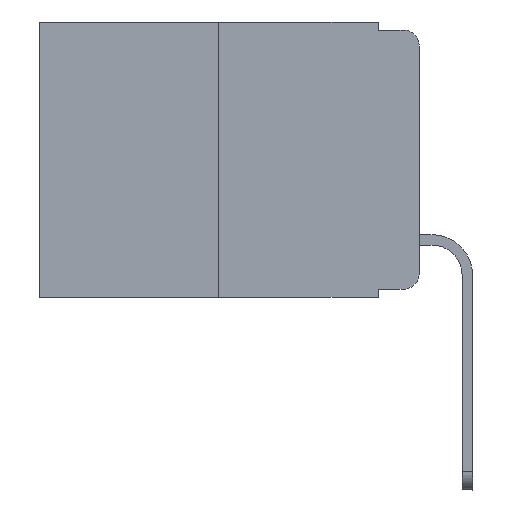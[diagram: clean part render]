
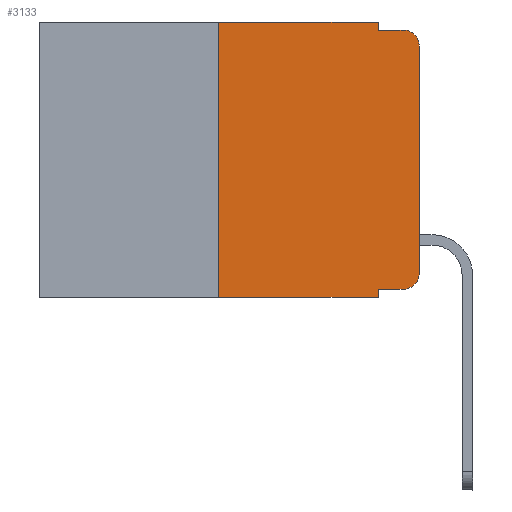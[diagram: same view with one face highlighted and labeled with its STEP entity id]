
A CAD part, left-side view. The second image highlights one B-rep face of the part: STEP entity #3133.
In plain terms, the highlighted planar face has unit normal (-1, 0, 0).
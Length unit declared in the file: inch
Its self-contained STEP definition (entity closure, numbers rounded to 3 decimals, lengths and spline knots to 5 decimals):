
#515 = DIRECTION ( 'NONE',  ( 1., 0., 0. ) ) ;
#656 = DIRECTION ( 'NONE',  ( -1., 0., 0. ) ) ;
#738 = VERTEX_POINT ( 'NONE', #8923 ) ;
#1302 = VECTOR ( 'NONE', #2873, 39.37008 ) ;
#1742 = ORIENTED_EDGE ( 'NONE', *, *, #2177, .F. ) ;
#1848 = CARTESIAN_POINT ( 'NONE',  ( 0., 0.051, 0. ) ) ;
#1941 = ORIENTED_EDGE ( 'NONE', *, *, #5974, .F. ) ;
#1996 = ORIENTED_EDGE ( 'NONE', *, *, #6174, .F. ) ;
#2177 = EDGE_CURVE ( 'NONE', #8845, #738, #9205, .T. ) ;
#2179 = CARTESIAN_POINT ( 'NONE',  ( 0., 0.25, -0.343 ) ) ;
#2196 = EDGE_CURVE ( 'NONE', #9051, #10114, #7529, .T. ) ;
#2361 = CARTESIAN_POINT ( 'NONE',  ( 0., 0.25, 0. ) ) ;
#2462 = AXIS2_PLACEMENT_3D ( 'NONE', #6807, #656, #8802 ) ;
#2551 = ORIENTED_EDGE ( 'NONE', *, *, #8033, .F. ) ;
#2873 = DIRECTION ( 'NONE',  ( 0., -1., 0. ) ) ;
#3044 = EDGE_CURVE ( 'NONE', #10114, #738, #8466, .T. ) ;
#3133 = ADVANCED_FACE ( 'NONE', ( #9075 ), #5826, .F. ) ;
#3138 = VERTEX_POINT ( 'NONE', #8938 ) ;
#3231 = VERTEX_POINT ( 'NONE', #10096 ) ;
#3804 = VERTEX_POINT ( 'NONE', #2179 ) ;
#4222 = CARTESIAN_POINT ( 'NONE',  ( 0., 0.02, -0.313 ) ) ;
#4401 = DIRECTION ( 'NONE',  ( 0., 0., 1. ) ) ;
#4646 = ORIENTED_EDGE ( 'NONE', *, *, #10714, .T. ) ;
#5015 = VERTEX_POINT ( 'NONE', #7576 ) ;
#5165 = DIRECTION ( 'NONE',  ( 0., 0., -1. ) ) ;
#5441 = VECTOR ( 'NONE', #5165, 39.37008 ) ;
#5453 = VECTOR ( 'NONE', #4401, 39.37008 ) ;
#5532 = CARTESIAN_POINT ( 'NONE',  ( 0., 0.051, -0.333 ) ) ;
#5826 = PLANE ( 'NONE',  #11360 ) ;
#5919 = LINE ( 'NONE', #10426, #5441 ) ;
#5974 = EDGE_CURVE ( 'NONE', #7213, #3231, #6970, .T. ) ;
#6174 = EDGE_CURVE ( 'NONE', #5015, #6857, #5919, .T. ) ;
#6487 = CARTESIAN_POINT ( 'NONE',  ( 0., 0., 0. ) ) ;
#6576 = LINE ( 'NONE', #5532, #11339 ) ;
#6732 = ORIENTED_EDGE ( 'NONE', *, *, #2196, .T. ) ;
#6751 = ORIENTED_EDGE ( 'NONE', *, *, #3044, .T. ) ;
#6807 = CARTESIAN_POINT ( 'NONE',  ( 0., 0.02, -0.03 ) ) ;
#6857 = VERTEX_POINT ( 'NONE', #8801 ) ;
#6858 = CARTESIAN_POINT ( 'NONE',  ( 0., 0., -0.03 ) ) ;
#6970 = LINE ( 'NONE', #13026, #13044 ) ;
#7167 = DIRECTION ( 'NONE',  ( 0., 0., -1. ) ) ;
#7213 = VERTEX_POINT ( 'NONE', #10994 ) ;
#7415 = DIRECTION ( 'NONE',  ( -1., 0., 0. ) ) ;
#7489 = ORIENTED_EDGE ( 'NONE', *, *, #10015, .T. ) ;
#7529 = LINE ( 'NONE', #6487, #9989 ) ;
#7560 = VECTOR ( 'NONE', #10317, 39.37008 ) ;
#7576 = CARTESIAN_POINT ( 'NONE',  ( 0., 0.051, -0.333 ) ) ;
#8033 = EDGE_CURVE ( 'NONE', #3231, #8845, #13486, .T. ) ;
#8180 = CARTESIAN_POINT ( 'NONE',  ( 0., 0.051, -0.01 ) ) ;
#8466 = CIRCLE ( 'NONE', #2462, 0.02 ) ;
#8619 = EDGE_LOOP ( 'NONE', ( #6732, #6751, #1742, #2551, #1941, #11229, #4646, #1996, #10237, #7489 ) ) ;
#8628 = CIRCLE ( 'NONE', #11059, 0.02 ) ;
#8801 = CARTESIAN_POINT ( 'NONE',  ( 0., 0.051, -0.343 ) ) ;
#8802 = DIRECTION ( 'NONE',  ( 0., 0., -1. ) ) ;
#8845 = VERTEX_POINT ( 'NONE', #9749 ) ;
#8923 = CARTESIAN_POINT ( 'NONE',  ( 0., 0.02, -0.01 ) ) ;
#8938 = CARTESIAN_POINT ( 'NONE',  ( 0., 0.02, -0.333 ) ) ;
#9006 = DIRECTION ( 'NONE',  ( 0., 0., -1. ) ) ;
#9051 = VERTEX_POINT ( 'NONE', #10518 ) ;
#9075 = FACE_OUTER_BOUND ( 'NONE', #8619, .T. ) ;
#9205 = LINE ( 'NONE', #8180, #7560 ) ;
#9254 = LINE ( 'NONE', #12406, #1302 ) ;
#9551 = DIRECTION ( 'NONE',  ( 0., 0., -1. ) ) ;
#9749 = CARTESIAN_POINT ( 'NONE',  ( 0., 0.051, -0.01 ) ) ;
#9812 = DIRECTION ( 'NONE',  ( 0., 0., 1. ) ) ;
#9989 = VECTOR ( 'NONE', #9812, 39.37008 ) ;
#10015 = EDGE_CURVE ( 'NONE', #3138, #9051, #8628, .T. ) ;
#10096 = CARTESIAN_POINT ( 'NONE',  ( 0., 0.051, 0. ) ) ;
#10114 = VERTEX_POINT ( 'NONE', #6858 ) ;
#10237 = ORIENTED_EDGE ( 'NONE', *, *, #11321, .T. ) ;
#10317 = DIRECTION ( 'NONE',  ( 0., -1., 0. ) ) ;
#10426 = CARTESIAN_POINT ( 'NONE',  ( 0., 0.051, 0. ) ) ;
#10518 = CARTESIAN_POINT ( 'NONE',  ( 0., 0., -0.313 ) ) ;
#10708 = LINE ( 'NONE', #2361, #5453 ) ;
#10714 = EDGE_CURVE ( 'NONE', #3804, #6857, #9254, .T. ) ;
#10994 = CARTESIAN_POINT ( 'NONE',  ( 0., 0.25, 0. ) ) ;
#11053 = DIRECTION ( 'NONE',  ( 0., -1., 0. ) ) ;
#11059 = AXIS2_PLACEMENT_3D ( 'NONE', #4222, #7415, #9551 ) ;
#11229 = ORIENTED_EDGE ( 'NONE', *, *, #13539, .F. ) ;
#11321 = EDGE_CURVE ( 'NONE', #5015, #3138, #6576, .T. ) ;
#11339 = VECTOR ( 'NONE', #12905, 39.37008 ) ;
#11360 = AXIS2_PLACEMENT_3D ( 'NONE', #13323, #515, #9006 ) ;
#12084 = VECTOR ( 'NONE', #7167, 39.37008 ) ;
#12406 = CARTESIAN_POINT ( 'NONE',  ( 0., 0.473, -0.343 ) ) ;
#12905 = DIRECTION ( 'NONE',  ( 0., -1., 0. ) ) ;
#13026 = CARTESIAN_POINT ( 'NONE',  ( 0., 0.473, 0. ) ) ;
#13044 = VECTOR ( 'NONE', #11053, 39.37008 ) ;
#13323 = CARTESIAN_POINT ( 'NONE',  ( 0., 0.473, 0. ) ) ;
#13486 = LINE ( 'NONE', #1848, #12084 ) ;
#13539 = EDGE_CURVE ( 'NONE', #3804, #7213, #10708, .T. ) ;
